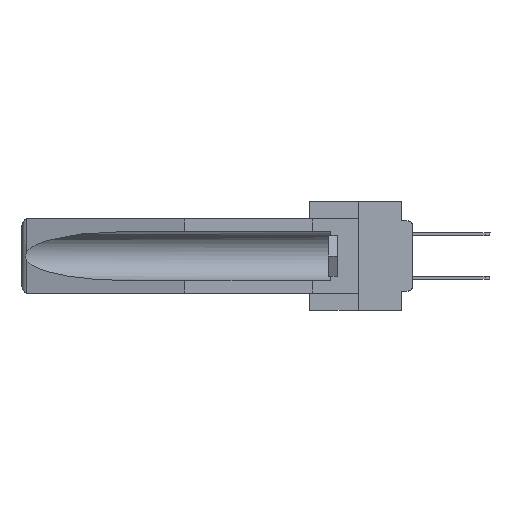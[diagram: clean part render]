
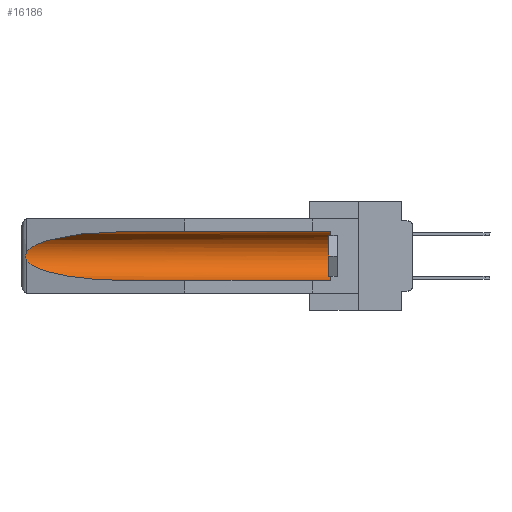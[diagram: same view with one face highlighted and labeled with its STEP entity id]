
A CAD part, left-side view. The second image highlights one B-rep face of the part: STEP entity #16186.
In plain terms, the highlighted cylindrical face has radius 2.857 mm (diameter 5.715 mm), a partial arc.
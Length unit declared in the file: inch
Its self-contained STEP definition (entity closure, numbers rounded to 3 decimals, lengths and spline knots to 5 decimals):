
#84 = AXIS2_PLACEMENT_3D ( 'NONE', #12027, #1715, #29170 ) ;
#141 = EDGE_CURVE ( 'NONE', #7359, #12776, #3287, .T. ) ;
#787 = ORIENTED_EDGE ( 'NONE', *, *, #141, .T. ) ;
#926 = CARTESIAN_POINT ( 'NONE',  ( 0.155, 1.07973, -0.059 ) ) ;
#1715 = DIRECTION ( 'NONE',  ( 0., -1., 0. ) ) ;
#3064 = EDGE_CURVE ( 'NONE', #22662, #26198, #5355, .T. ) ;
#3287 =( BOUNDED_CURVE ( )  B_SPLINE_CURVE ( 3, ( #19174, #32017, #4534, #32503 ),
 .UNSPECIFIED., .F., .F. ) 
 B_SPLINE_CURVE_WITH_KNOTS ( ( 4, 4 ),
 ( 0.1948, 1.5708 ),
 .UNSPECIFIED. ) 
 CURVE ( )  GEOMETRIC_REPRESENTATION_ITEM ( )  RATIONAL_B_SPLINE_CURVE ( ( 1., 0.848, 0.848, 1. ) ) 
 REPRESENTATION_ITEM ( '' )  );
#3824 = ORIENTED_EDGE ( 'NONE', *, *, #11216, .T. ) ;
#4534 = CARTESIAN_POINT ( 'NONE',  ( 0.21114, 1.30732, -0.284 ) ) ;
#4874 = VERTEX_POINT ( 'NONE', #5603 ) ;
#4897 = DIRECTION ( 'NONE',  ( 0., 1., 0. ) ) ;
#5355 = LINE ( 'NONE', #20164, #7246 ) ;
#5603 = CARTESIAN_POINT ( 'NONE',  ( 0.155, 0.126, -0.284 ) ) ;
#6066 = CARTESIAN_POINT ( 'NONE',  ( 0.21114, 1.30732, -0.059 ) ) ;
#6232 = DIRECTION ( 'NONE',  ( 0., 0., 1. ) ) ;
#6242 = EDGE_CURVE ( 'NONE', #21643, #7359, #18035, .T. ) ;
#6791 = ORIENTED_EDGE ( 'NONE', *, *, #19251, .T. ) ;
#7035 = CARTESIAN_POINT ( 'NONE',  ( 0.26537, 1.52718, -0.19328 ) ) ;
#7246 = VECTOR ( 'NONE', #10688, 39.37008 ) ;
#7359 = VERTEX_POINT ( 'NONE', #18718 ) ;
#8391 = CARTESIAN_POINT ( 'NONE',  ( 0.155, 0.126, -0.059 ) ) ;
#9384 = DIRECTION ( 'NONE',  ( 0., 1., 0. ) ) ;
#9702 = CARTESIAN_POINT ( 'NONE',  ( 0.26597, 1.5296, -0.19026 ) ) ;
#10688 = DIRECTION ( 'NONE',  ( 0., 1., 0. ) ) ;
#11216 = EDGE_CURVE ( 'NONE', #26198, #21643, #32651, .T. ) ;
#11413 = FACE_OUTER_BOUND ( 'NONE', #24129, .T. ) ;
#11576 = CARTESIAN_POINT ( 'NONE',  ( 0.155, -0.30754, -0.1715 ) ) ;
#12027 = CARTESIAN_POINT ( 'NONE',  ( 0.155, 0.126, -0.1715 ) ) ;
#12776 = VERTEX_POINT ( 'NONE', #27228 ) ;
#14463 = CIRCLE ( 'NONE', #84, 0.1125 ) ;
#14885 = CARTESIAN_POINT ( 'NONE',  ( 0.26655, 1.53094, -0.18657 ) ) ;
#16186 = ADVANCED_FACE ( 'NONE', ( #11413 ), #29542, .F. ) ;
#17376 = CARTESIAN_POINT ( 'NONE',  ( 0.26537, 1.52718, -0.14972 ) ) ;
#17534 = CARTESIAN_POINT ( 'NONE',  ( 0.2675, 1.53308, -0.16763 ) ) ;
#18035 = B_SPLINE_CURVE_WITH_KNOTS ( 'NONE', 3,
 ( #17376, #30191, #30035, #24708, #17534, #22358, #27696, #14885, #9702, #7035 ),
 .UNSPECIFIED., .F., .F.,
 ( 4, 2, 2, 2, 4 ),
 ( 0., 0.00029, 0.00058, 0.00087, 0.00117 ),
 .UNSPECIFIED. ) ;
#18350 = VECTOR ( 'NONE', #4897, 39.37008 ) ;
#18718 = CARTESIAN_POINT ( 'NONE',  ( 0.26537, 1.52718, -0.19328 ) ) ;
#19174 = CARTESIAN_POINT ( 'NONE',  ( 0.26537, 1.52718, -0.19328 ) ) ;
#19251 = EDGE_CURVE ( 'NONE', #4874, #22662, #14463, .T. ) ;
#20164 = CARTESIAN_POINT ( 'NONE',  ( 0.155, -0.30754, -0.059 ) ) ;
#21378 = CARTESIAN_POINT ( 'NONE',  ( 0.25451, 1.48313, -0.09465 ) ) ;
#21643 = VERTEX_POINT ( 'NONE', #24918 ) ;
#21661 = CARTESIAN_POINT ( 'NONE',  ( 0.155, 1.07973, -0.059 ) ) ;
#22358 = CARTESIAN_POINT ( 'NONE',  ( 0.2675, 1.53308, -0.17534 ) ) ;
#22662 = VERTEX_POINT ( 'NONE', #8391 ) ;
#24056 = CARTESIAN_POINT ( 'NONE',  ( 0.26537, 1.52718, -0.14972 ) ) ;
#24129 = EDGE_LOOP ( 'NONE', ( #3824, #24143, #787, #24931, #6791, #25055 ) ) ;
#24141 = EDGE_CURVE ( 'NONE', #4874, #12776, #25206, .T. ) ;
#24143 = ORIENTED_EDGE ( 'NONE', *, *, #6242, .T. ) ;
#24708 = CARTESIAN_POINT ( 'NONE',  ( 0.2673, 1.5327, -0.16383 ) ) ;
#24918 = CARTESIAN_POINT ( 'NONE',  ( 0.26537, 1.52718, -0.14972 ) ) ;
#24931 = ORIENTED_EDGE ( 'NONE', *, *, #24141, .F. ) ;
#25055 = ORIENTED_EDGE ( 'NONE', *, *, #3064, .T. ) ;
#25206 = LINE ( 'NONE', #32726, #18350 ) ;
#26198 = VERTEX_POINT ( 'NONE', #21661 ) ;
#27228 = CARTESIAN_POINT ( 'NONE',  ( 0.155, 1.07973, -0.284 ) ) ;
#27696 = CARTESIAN_POINT ( 'NONE',  ( 0.2673, 1.53269, -0.17917 ) ) ;
#29023 = AXIS2_PLACEMENT_3D ( 'NONE', #11576, #9384, #6232 ) ;
#29170 = DIRECTION ( 'NONE',  ( 0., 0., 1. ) ) ;
#29542 = CYLINDRICAL_SURFACE ( 'NONE', #29023, 0.1125 ) ;
#30035 = CARTESIAN_POINT ( 'NONE',  ( 0.26654, 1.53092, -0.15636 ) ) ;
#30191 = CARTESIAN_POINT ( 'NONE',  ( 0.26597, 1.52961, -0.15275 ) ) ;
#32017 = CARTESIAN_POINT ( 'NONE',  ( 0.25451, 1.48313, -0.24835 ) ) ;
#32503 = CARTESIAN_POINT ( 'NONE',  ( 0.155, 1.07973, -0.284 ) ) ;
#32651 =( BOUNDED_CURVE ( )  B_SPLINE_CURVE ( 3, ( #926, #6066, #21378, #24056 ),
 .UNSPECIFIED., .F., .F. ) 
 B_SPLINE_CURVE_WITH_KNOTS ( ( 4, 4 ),
 ( 4.71239, 6.08839 ),
 .UNSPECIFIED. ) 
 CURVE ( )  GEOMETRIC_REPRESENTATION_ITEM ( )  RATIONAL_B_SPLINE_CURVE ( ( 1., 0.848, 0.848, 1. ) ) 
 REPRESENTATION_ITEM ( '' )  );
#32726 = CARTESIAN_POINT ( 'NONE',  ( 0.155, -0.30754, -0.284 ) ) ;
